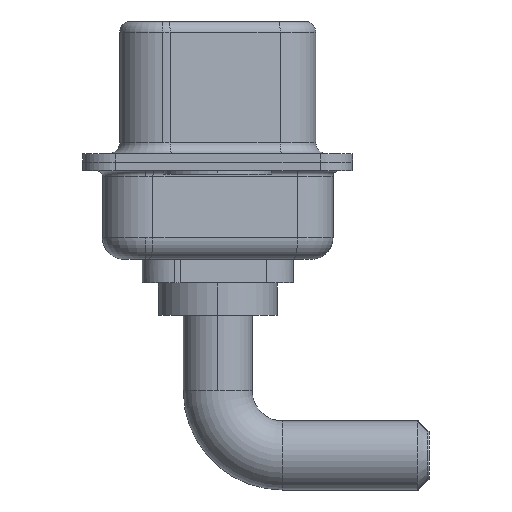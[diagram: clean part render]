
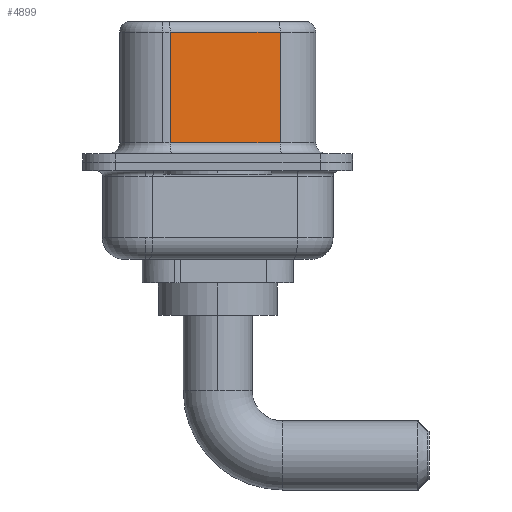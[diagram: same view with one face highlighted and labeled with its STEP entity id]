
A CAD part, left-side view. The second image highlights one B-rep face of the part: STEP entity #4899.
In plain terms, the highlighted planar face has unit normal (-0.985, -0.174, 0).
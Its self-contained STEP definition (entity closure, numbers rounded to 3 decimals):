
#366 = DIRECTION ( 'NONE',  ( 0.174, -0.985, 0. ) ) ;
#429 = CARTESIAN_POINT ( 'NONE',  ( 4.58, -2.897, 0.9 ) ) ;
#1126 = LINE ( 'NONE', #429, #11674 ) ;
#1227 = VECTOR ( 'NONE', #10509, 1000. ) ;
#1309 = DIRECTION ( 'NONE',  ( 0., 0., -1. ) ) ;
#1830 = EDGE_CURVE ( 'NONE', #8591, #12248, #10907, .T. ) ;
#2065 = CARTESIAN_POINT ( 'NONE',  ( 4.58, -2.897, 6.52 ) ) ;
#2166 = CARTESIAN_POINT ( 'NONE',  ( 3.68, 2.203, 6.02 ) ) ;
#2334 = CARTESIAN_POINT ( 'NONE',  ( 4.58, -2.897, 0.9 ) ) ;
#4183 = EDGE_CURVE ( 'NONE', #10227, #10072, #7631, .T. ) ;
#4468 = EDGE_LOOP ( 'NONE', ( #5778, #10885, #4972, #10673 ) ) ;
#4663 = DIRECTION ( 'NONE',  ( -0.174, 0.985, 0. ) ) ;
#4892 = EDGE_CURVE ( 'NONE', #8591, #10227, #5683, .T. ) ;
#4899 = ADVANCED_FACE ( 'NONE', ( #8606 ), #7535, .F. ) ;
#4972 = ORIENTED_EDGE ( 'NONE', *, *, #4183, .T. ) ;
#5683 = LINE ( 'NONE', #7778, #6570 ) ;
#5778 = ORIENTED_EDGE ( 'NONE', *, *, #1830, .F. ) ;
#6570 = VECTOR ( 'NONE', #4663, 1000. ) ;
#6677 = CARTESIAN_POINT ( 'NONE',  ( 3.68, 2.203, 6.52 ) ) ;
#6724 = CARTESIAN_POINT ( 'NONE',  ( 3.68, 2.203, 0.9 ) ) ;
#6832 = DIRECTION ( 'NONE',  ( -0.174, 0.985, 0. ) ) ;
#7258 = CARTESIAN_POINT ( 'NONE',  ( 4.58, -2.897, 6.02 ) ) ;
#7535 = PLANE ( 'NONE',  #9180 ) ;
#7631 = LINE ( 'NONE', #6677, #1227 ) ;
#7778 = CARTESIAN_POINT ( 'NONE',  ( 4.58, -2.897, 6.02 ) ) ;
#8591 = VERTEX_POINT ( 'NONE', #7258 ) ;
#8606 = FACE_OUTER_BOUND ( 'NONE', #4468, .T. ) ;
#9180 = AXIS2_PLACEMENT_3D ( 'NONE', #9536, #11633, #6832 ) ;
#9502 = VECTOR ( 'NONE', #1309, 1000. ) ;
#9536 = CARTESIAN_POINT ( 'NONE',  ( 4.58, -2.897, 6.52 ) ) ;
#10072 = VERTEX_POINT ( 'NONE', #6724 ) ;
#10227 = VERTEX_POINT ( 'NONE', #2166 ) ;
#10509 = DIRECTION ( 'NONE',  ( 0., 0., -1. ) ) ;
#10673 = ORIENTED_EDGE ( 'NONE', *, *, #12325, .T. ) ;
#10885 = ORIENTED_EDGE ( 'NONE', *, *, #4892, .T. ) ;
#10907 = LINE ( 'NONE', #2065, #9502 ) ;
#11633 = DIRECTION ( 'NONE',  ( 0.985, 0.174, 0. ) ) ;
#11674 = VECTOR ( 'NONE', #366, 1000. ) ;
#12248 = VERTEX_POINT ( 'NONE', #2334 ) ;
#12325 = EDGE_CURVE ( 'NONE', #10072, #12248, #1126, .T. ) ;
